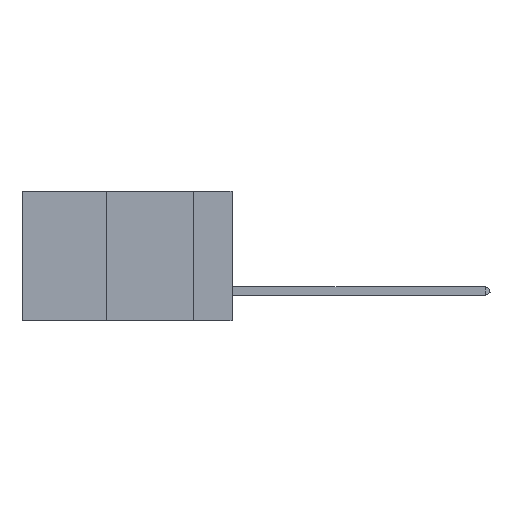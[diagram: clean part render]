
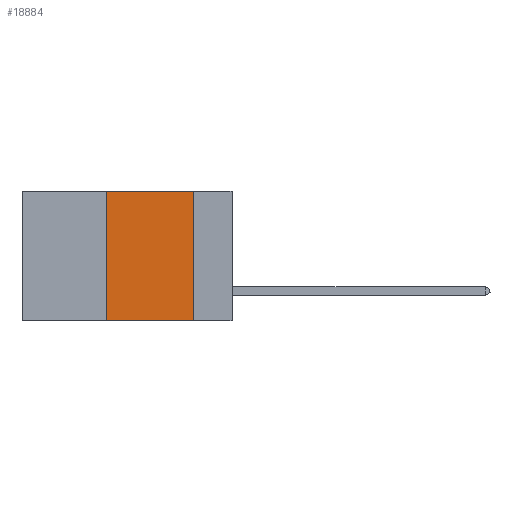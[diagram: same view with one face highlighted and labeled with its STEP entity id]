
A CAD part, left-side view. The second image highlights one B-rep face of the part: STEP entity #18884.
In plain terms, the highlighted planar face has unit normal (-1, 0, 0).
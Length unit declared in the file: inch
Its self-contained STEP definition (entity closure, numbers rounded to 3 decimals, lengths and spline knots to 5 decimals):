
#644 = VERTEX_POINT ( 'NONE', #15156 ) ;
#755 = LINE ( 'NONE', #14068, #3997 ) ;
#1225 = ORIENTED_EDGE ( 'NONE', *, *, #17170, .T. ) ;
#1819 = LINE ( 'NONE', #8643, #19279 ) ;
#2144 = EDGE_CURVE ( 'NONE', #10485, #18338, #19087, .T. ) ;
#2711 = ORIENTED_EDGE ( 'NONE', *, *, #15332, .F. ) ;
#3300 = EDGE_CURVE ( 'NONE', #644, #8506, #1819, .T. ) ;
#3997 = VECTOR ( 'NONE', #7169, 39.37008 ) ;
#4291 = VECTOR ( 'NONE', #19480, 39.37008 ) ;
#5048 = CARTESIAN_POINT ( 'NONE',  ( 0., 0.6, 0. ) ) ;
#6190 = CARTESIAN_POINT ( 'NONE',  ( 0., 0.11, -0.37 ) ) ;
#6626 = VECTOR ( 'NONE', #7254, 39.37008 ) ;
#6793 = DIRECTION ( 'NONE',  ( 0., 0., -1. ) ) ;
#7169 = DIRECTION ( 'NONE',  ( 0., -1., 0. ) ) ;
#7254 = DIRECTION ( 'NONE',  ( 0., -1., 0. ) ) ;
#8506 = VERTEX_POINT ( 'NONE', #6190 ) ;
#8643 = CARTESIAN_POINT ( 'NONE',  ( 0., 0.11, 0. ) ) ;
#9826 = FACE_OUTER_BOUND ( 'NONE', #12113, .T. ) ;
#10485 = VERTEX_POINT ( 'NONE', #16627 ) ;
#11161 = CARTESIAN_POINT ( 'NONE',  ( 0., 0.36, 0. ) ) ;
#12113 = EDGE_LOOP ( 'NONE', ( #21866, #2711, #15470, #1225 ) ) ;
#12144 = DIRECTION ( 'NONE',  ( 0., 0., -1. ) ) ;
#14068 = CARTESIAN_POINT ( 'NONE',  ( 0., 0.6, 0. ) ) ;
#14739 = CARTESIAN_POINT ( 'NONE',  ( 0., 0.36, 0. ) ) ;
#15156 = CARTESIAN_POINT ( 'NONE',  ( 0., 0.11, 0. ) ) ;
#15332 = EDGE_CURVE ( 'NONE', #18338, #644, #755, .T. ) ;
#15402 = PLANE ( 'NONE',  #17493 ) ;
#15470 = ORIENTED_EDGE ( 'NONE', *, *, #2144, .F. ) ;
#15536 = LINE ( 'NONE', #22125, #6626 ) ;
#16627 = CARTESIAN_POINT ( 'NONE',  ( 0., 0.36, -0.37 ) ) ;
#17170 = EDGE_CURVE ( 'NONE', #10485, #8506, #15536, .T. ) ;
#17493 = AXIS2_PLACEMENT_3D ( 'NONE', #5048, #20625, #6793 ) ;
#18338 = VERTEX_POINT ( 'NONE', #14739 ) ;
#18884 = ADVANCED_FACE ( 'NONE', ( #9826 ), #15402, .F. ) ;
#19087 = LINE ( 'NONE', #11161, #4291 ) ;
#19279 = VECTOR ( 'NONE', #12144, 39.37008 ) ;
#19480 = DIRECTION ( 'NONE',  ( 0., 0., 1. ) ) ;
#20625 = DIRECTION ( 'NONE',  ( 1., 0., 0. ) ) ;
#21866 = ORIENTED_EDGE ( 'NONE', *, *, #3300, .F. ) ;
#22125 = CARTESIAN_POINT ( 'NONE',  ( 0., 0.6, -0.37 ) ) ;
